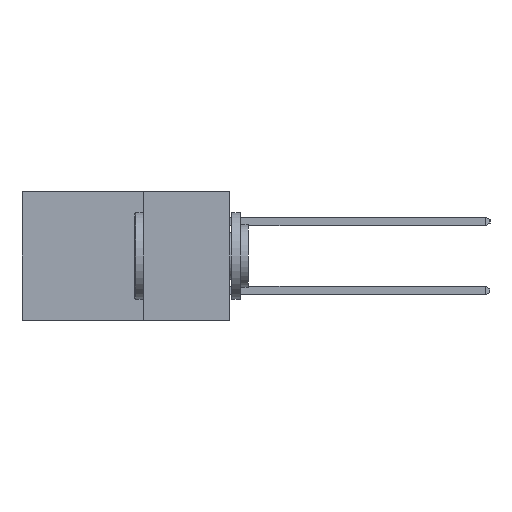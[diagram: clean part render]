
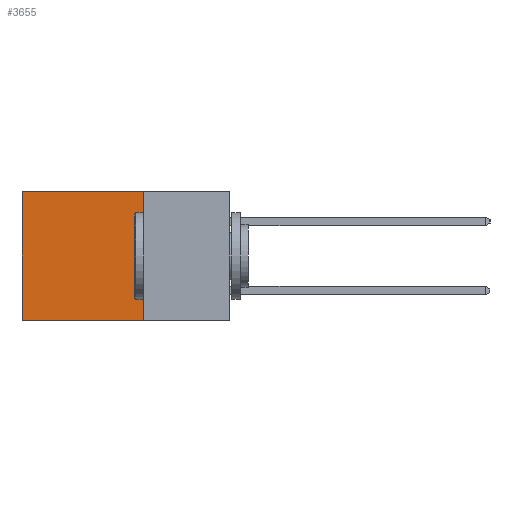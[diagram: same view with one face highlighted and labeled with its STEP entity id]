
A CAD part, left-side view. The second image highlights one B-rep face of the part: STEP entity #3655.
In plain terms, the highlighted planar face has unit normal (-1, 0, 0).
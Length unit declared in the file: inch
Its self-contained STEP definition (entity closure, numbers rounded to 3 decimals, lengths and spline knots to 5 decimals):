
#225 = VERTEX_POINT ( 'NONE', #2069 ) ;
#322 = AXIS2_PLACEMENT_3D ( 'NONE', #4648, #5564, #5485 ) ;
#1155 = EDGE_CURVE ( 'NONE', #225, #2189, #2297, .T. ) ;
#1811 = CARTESIAN_POINT ( 'NONE',  ( 0.298, 0.6, 0. ) ) ;
#2069 = CARTESIAN_POINT ( 'NONE',  ( 0.298, 0.25, 0. ) ) ;
#2082 = ORIENTED_EDGE ( 'NONE', *, *, #7378, .T. ) ;
#2127 = CARTESIAN_POINT ( 'NONE',  ( 0.298, 0.6, -0.37 ) ) ;
#2166 = VECTOR ( 'NONE', #9085, 39.37008 ) ;
#2189 = VERTEX_POINT ( 'NONE', #1811 ) ;
#2297 = LINE ( 'NONE', #12348, #4862 ) ;
#2381 = CARTESIAN_POINT ( 'NONE',  ( 0.298, 0.6, 0. ) ) ;
#2406 = LINE ( 'NONE', #4035, #12161 ) ;
#2490 = VERTEX_POINT ( 'NONE', #8285 ) ;
#3004 = FACE_OUTER_BOUND ( 'NONE', #8623, .T. ) ;
#3207 = EDGE_CURVE ( 'NONE', #2490, #5152, #2406, .T. ) ;
#3516 = EDGE_CURVE ( 'NONE', #225, #2490, #11751, .T. ) ;
#3655 = ADVANCED_FACE ( 'NONE', ( #3004 ), #4930, .F. ) ;
#3830 = LINE ( 'NONE', #2381, #2166 ) ;
#4035 = CARTESIAN_POINT ( 'NONE',  ( 0.298, 0.25, -0.37 ) ) ;
#4264 = CARTESIAN_POINT ( 'NONE',  ( 0.298, 0.25, 0. ) ) ;
#4500 = DIRECTION ( 'NONE',  ( 0., 0., -1. ) ) ;
#4648 = CARTESIAN_POINT ( 'NONE',  ( 0.298, 0.25, 0. ) ) ;
#4862 = VECTOR ( 'NONE', #11992, 39.37008 ) ;
#4930 = PLANE ( 'NONE',  #322 ) ;
#5152 = VERTEX_POINT ( 'NONE', #2127 ) ;
#5485 = DIRECTION ( 'NONE',  ( 0., 0., -1. ) ) ;
#5564 = DIRECTION ( 'NONE',  ( 1., 0., 0. ) ) ;
#7378 = EDGE_CURVE ( 'NONE', #2189, #5152, #3830, .T. ) ;
#7854 = ORIENTED_EDGE ( 'NONE', *, *, #1155, .T. ) ;
#8285 = CARTESIAN_POINT ( 'NONE',  ( 0.298, 0.25, -0.37 ) ) ;
#8623 = EDGE_LOOP ( 'NONE', ( #2082, #11803, #12235, #7854 ) ) ;
#9085 = DIRECTION ( 'NONE',  ( 0., 0., -1. ) ) ;
#9275 = VECTOR ( 'NONE', #4500, 39.37008 ) ;
#11751 = LINE ( 'NONE', #4264, #9275 ) ;
#11803 = ORIENTED_EDGE ( 'NONE', *, *, #3207, .F. ) ;
#11992 = DIRECTION ( 'NONE',  ( 0., 1., 0. ) ) ;
#12161 = VECTOR ( 'NONE', #12226, 39.37008 ) ;
#12226 = DIRECTION ( 'NONE',  ( 0., 1., 0. ) ) ;
#12235 = ORIENTED_EDGE ( 'NONE', *, *, #3516, .F. ) ;
#12348 = CARTESIAN_POINT ( 'NONE',  ( 0.298, 0.25, 0. ) ) ;
